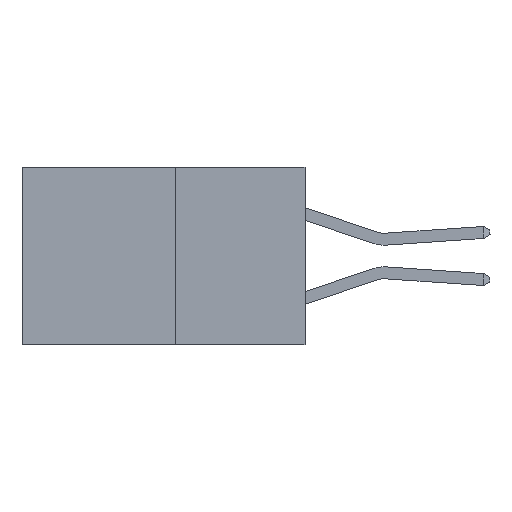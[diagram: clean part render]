
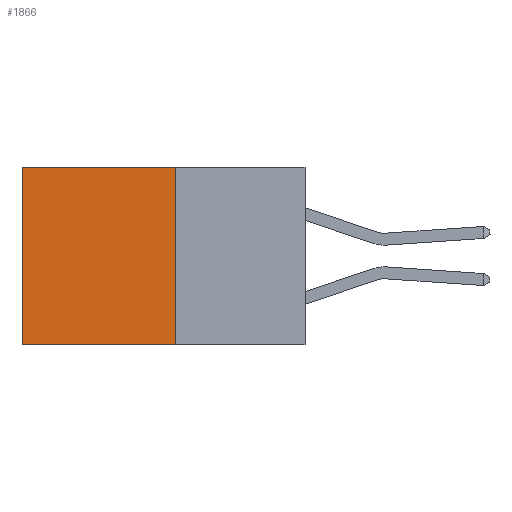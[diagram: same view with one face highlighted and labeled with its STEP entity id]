
A CAD part, left-side view. The second image highlights one B-rep face of the part: STEP entity #1866.
In plain terms, the highlighted planar face has unit normal (-1, 0, 0).
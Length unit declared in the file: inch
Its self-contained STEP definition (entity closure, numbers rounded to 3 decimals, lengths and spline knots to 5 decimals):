
#164 = LINE ( 'NONE', #3871, #3569 ) ;
#580 = CARTESIAN_POINT ( 'NONE',  ( 0.277, 0.27, -0.37 ) ) ;
#585 = VERTEX_POINT ( 'NONE', #2579 ) ;
#588 = ORIENTED_EDGE ( 'NONE', *, *, #3334, .F. ) ;
#651 = CARTESIAN_POINT ( 'NONE',  ( 0.277, 0.59, -0.37 ) ) ;
#1049 = LINE ( 'NONE', #1252, #4468 ) ;
#1102 = EDGE_CURVE ( 'NONE', #585, #7116, #8338, .T. ) ;
#1120 = VERTEX_POINT ( 'NONE', #5557 ) ;
#1252 = CARTESIAN_POINT ( 'NONE',  ( 0.277, 0.59, -0.37 ) ) ;
#1255 = VECTOR ( 'NONE', #6085, 39.37008 ) ;
#1335 = DIRECTION ( 'NONE',  ( 0., 0., -1. ) ) ;
#1493 = EDGE_CURVE ( 'NONE', #7116, #2397, #1049, .T. ) ;
#1839 = CARTESIAN_POINT ( 'NONE',  ( 0.277, 0.27, 0. ) ) ;
#1866 = ADVANCED_FACE ( 'NONE', ( #2312 ), #7447, .F. ) ;
#1950 = AXIS2_PLACEMENT_3D ( 'NONE', #580, #7544, #4191 ) ;
#2293 = DIRECTION ( 'NONE',  ( 0., 0., -1. ) ) ;
#2312 = FACE_OUTER_BOUND ( 'NONE', #4794, .T. ) ;
#2397 = VERTEX_POINT ( 'NONE', #651 ) ;
#2579 = CARTESIAN_POINT ( 'NONE',  ( 0.277, 0.27, 0. ) ) ;
#3238 = LINE ( 'NONE', #5765, #6675 ) ;
#3334 = EDGE_CURVE ( 'NONE', #1120, #2397, #3238, .T. ) ;
#3427 = EDGE_CURVE ( 'NONE', #585, #1120, #164, .T. ) ;
#3569 = VECTOR ( 'NONE', #1335, 39.37008 ) ;
#3601 = ORIENTED_EDGE ( 'NONE', *, *, #1102, .T. ) ;
#3675 = DIRECTION ( 'NONE',  ( 0., 1., 0. ) ) ;
#3871 = CARTESIAN_POINT ( 'NONE',  ( 0.277, 0.27, -0.37 ) ) ;
#4191 = DIRECTION ( 'NONE',  ( 0., 0., -1. ) ) ;
#4468 = VECTOR ( 'NONE', #2293, 39.37008 ) ;
#4794 = EDGE_LOOP ( 'NONE', ( #6107, #588, #7567, #3601 ) ) ;
#5557 = CARTESIAN_POINT ( 'NONE',  ( 0.277, 0.27, -0.37 ) ) ;
#5765 = CARTESIAN_POINT ( 'NONE',  ( 0.277, 0.27, -0.37 ) ) ;
#6085 = DIRECTION ( 'NONE',  ( 0., 1., 0. ) ) ;
#6107 = ORIENTED_EDGE ( 'NONE', *, *, #1493, .T. ) ;
#6675 = VECTOR ( 'NONE', #3675, 39.37008 ) ;
#7116 = VERTEX_POINT ( 'NONE', #7571 ) ;
#7447 = PLANE ( 'NONE',  #1950 ) ;
#7544 = DIRECTION ( 'NONE',  ( 1., 0., 0. ) ) ;
#7567 = ORIENTED_EDGE ( 'NONE', *, *, #3427, .F. ) ;
#7571 = CARTESIAN_POINT ( 'NONE',  ( 0.277, 0.59, 0. ) ) ;
#8338 = LINE ( 'NONE', #1839, #1255 ) ;
